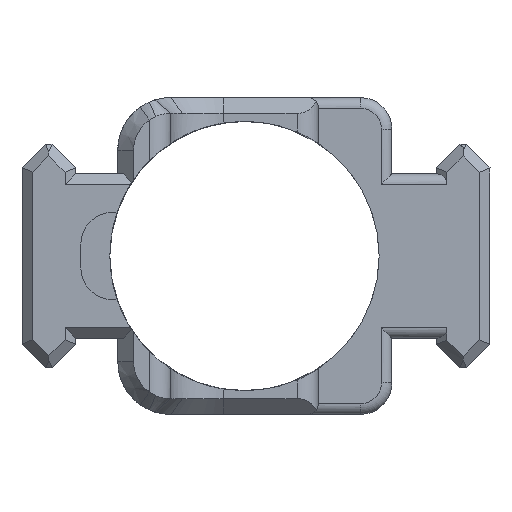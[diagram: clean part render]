
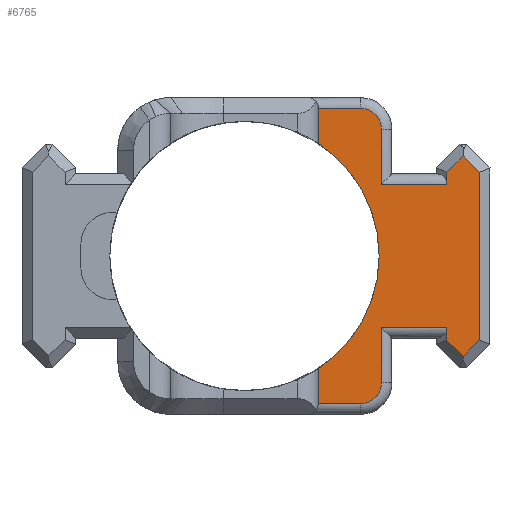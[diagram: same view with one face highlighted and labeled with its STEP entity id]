
A CAD part, left-side view. The second image highlights one B-rep face of the part: STEP entity #6765.
In plain terms, the highlighted planar face has unit normal (-1, 0, 0).
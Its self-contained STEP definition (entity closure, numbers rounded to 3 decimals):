
#152=CIRCLE('',#7203,12.75);
#161=CIRCLE('',#7226,2.);
#162=CIRCLE('',#7227,2.);
#275=FACE_OUTER_BOUND('',#668,.T.);
#668=EDGE_LOOP('',(#4912,#4913,#4914,#4915,#4916,#4917,#4918,#4919,#4920,
#4921,#4922,#4923,#4924,#4925,#4926,#4927,#4928,#4929));
#1260=LINE('',#10404,#2133);
#1261=LINE('',#10408,#2134);
#1264=LINE('',#10424,#2137);
#1268=LINE('',#10437,#2141);
#1269=LINE('',#10439,#2142);
#1270=LINE('',#10441,#2143);
#1271=LINE('',#10443,#2144);
#1272=LINE('',#10445,#2145);
#1273=LINE('',#10447,#2146);
#1274=LINE('',#10449,#2147);
#1275=LINE('',#10451,#2148);
#1276=LINE('',#10453,#2149);
#1277=LINE('',#10455,#2150);
#1278=LINE('',#10457,#2151);
#1279=LINE('',#10460,#2152);
#2133=VECTOR('',#8093,10.);
#2134=VECTOR('',#8098,10.);
#2137=VECTOR('',#8109,10.);
#2141=VECTOR('',#8123,10.);
#2142=VECTOR('',#8124,10.);
#2143=VECTOR('',#8125,10.);
#2144=VECTOR('',#8126,10.);
#2145=VECTOR('',#8127,10.);
#2146=VECTOR('',#8128,10.);
#2147=VECTOR('',#8129,10.);
#2148=VECTOR('',#8130,10.);
#2149=VECTOR('',#8131,10.);
#2150=VECTOR('',#8132,10.);
#2151=VECTOR('',#8133,10.);
#2152=VECTOR('',#8136,10.);
#2971=VERTEX_POINT('',#10185);
#2978=VERTEX_POINT('',#10219);
#2979=VERTEX_POINT('',#10221);
#3006=VERTEX_POINT('',#10406);
#3009=VERTEX_POINT('',#10418);
#3012=VERTEX_POINT('',#10434);
#3013=VERTEX_POINT('',#10436);
#3014=VERTEX_POINT('',#10438);
#3015=VERTEX_POINT('',#10440);
#3016=VERTEX_POINT('',#10442);
#3017=VERTEX_POINT('',#10444);
#3018=VERTEX_POINT('',#10446);
#3019=VERTEX_POINT('',#10448);
#3020=VERTEX_POINT('',#10450);
#3021=VERTEX_POINT('',#10452);
#3022=VERTEX_POINT('',#10454);
#3023=VERTEX_POINT('',#10456);
#3024=VERTEX_POINT('',#10458);
#3669=EDGE_CURVE('',#2979,#2978,#152,.T.);
#3701=EDGE_CURVE('',#2978,#2971,#1260,.T.);
#3703=EDGE_CURVE('',#3006,#2971,#1261,.T.);
#3709=EDGE_CURVE('',#3009,#2979,#1264,.T.);
#3714=EDGE_CURVE('',#3012,#3006,#161,.T.);
#3715=EDGE_CURVE('',#3013,#3012,#1268,.T.);
#3716=EDGE_CURVE('',#3014,#3013,#1269,.T.);
#3717=EDGE_CURVE('',#3015,#3014,#1270,.T.);
#3718=EDGE_CURVE('',#3016,#3015,#1271,.T.);
#3719=EDGE_CURVE('',#3017,#3016,#1272,.T.);
#3720=EDGE_CURVE('',#3018,#3017,#1273,.T.);
#3721=EDGE_CURVE('',#3019,#3018,#1274,.T.);
#3722=EDGE_CURVE('',#3020,#3019,#1275,.T.);
#3723=EDGE_CURVE('',#3021,#3020,#1276,.T.);
#3724=EDGE_CURVE('',#3022,#3021,#1277,.T.);
#3725=EDGE_CURVE('',#3023,#3022,#1278,.T.);
#3726=EDGE_CURVE('',#3024,#3023,#162,.T.);
#3727=EDGE_CURVE('',#3009,#3024,#1279,.T.);
#4912=ORIENTED_EDGE('',*,*,#3669,.T.);
#4913=ORIENTED_EDGE('',*,*,#3701,.T.);
#4914=ORIENTED_EDGE('',*,*,#3703,.F.);
#4915=ORIENTED_EDGE('',*,*,#3714,.F.);
#4916=ORIENTED_EDGE('',*,*,#3715,.F.);
#4917=ORIENTED_EDGE('',*,*,#3716,.F.);
#4918=ORIENTED_EDGE('',*,*,#3717,.F.);
#4919=ORIENTED_EDGE('',*,*,#3718,.F.);
#4920=ORIENTED_EDGE('',*,*,#3719,.F.);
#4921=ORIENTED_EDGE('',*,*,#3720,.F.);
#4922=ORIENTED_EDGE('',*,*,#3721,.F.);
#4923=ORIENTED_EDGE('',*,*,#3722,.F.);
#4924=ORIENTED_EDGE('',*,*,#3723,.F.);
#4925=ORIENTED_EDGE('',*,*,#3724,.F.);
#4926=ORIENTED_EDGE('',*,*,#3725,.F.);
#4927=ORIENTED_EDGE('',*,*,#3726,.F.);
#4928=ORIENTED_EDGE('',*,*,#3727,.F.);
#4929=ORIENTED_EDGE('',*,*,#3709,.T.);
#6403=PLANE('',#7225);
#6765=ADVANCED_FACE('',(#275),#6403,.T.);
#7203=AXIS2_PLACEMENT_3D('',#10222,#8058,#8059);
#7225=AXIS2_PLACEMENT_3D('',#10433,#8119,#8120);
#7226=AXIS2_PLACEMENT_3D('',#10435,#8121,#8122);
#7227=AXIS2_PLACEMENT_3D('',#10459,#8134,#8135);
#8058=DIRECTION('center_axis',(1.,0.,0.));
#8059=DIRECTION('ref_axis',(0.,-1.,0.));
#8093=DIRECTION('',(0.,0.,-1.));
#8098=DIRECTION('',(0.,1.,0.));
#8109=DIRECTION('',(0.,0.,-1.));
#8119=DIRECTION('center_axis',(-1.,0.,0.));
#8120=DIRECTION('ref_axis',(0.,-1.,0.));
#8121=DIRECTION('center_axis',(1.,0.,0.));
#8122=DIRECTION('ref_axis',(0.,-0.707,-0.707));
#8123=DIRECTION('',(0.,0.,-1.));
#8124=DIRECTION('',(0.,1.,0.));
#8125=DIRECTION('',(0.,0.,1.));
#8126=DIRECTION('',(0.,0.707,0.707));
#8127=DIRECTION('',(0.,0.707,-0.707));
#8128=DIRECTION('',(0.,0.,-1.));
#8129=DIRECTION('',(0.,-0.707,-0.707));
#8130=DIRECTION('',(0.,-0.707,0.707));
#8131=DIRECTION('',(0.,0.,1.));
#8132=DIRECTION('',(0.,-1.,0.));
#8133=DIRECTION('',(0.,0.,-1.));
#8134=DIRECTION('center_axis',(1.,0.,0.));
#8135=DIRECTION('ref_axis',(0.,-0.707,0.707));
#8136=DIRECTION('',(0.,-1.,0.));
#10185=CARTESIAN_POINT('',(-1.,86.015,1.));
#10219=CARTESIAN_POINT('',(-1.,86.015,4.334));
#10221=CARTESIAN_POINT('',(-1.,86.015,25.666));
#10222=CARTESIAN_POINT('Origin',(-1.,93.,15.));
#10404=CARTESIAN_POINT('',(-1.,86.015,0.));
#10406=CARTESIAN_POINT('',(-1.,82.03,1.));
#10408=CARTESIAN_POINT('',(-1.,101.5,1.));
#10418=CARTESIAN_POINT('',(-1.,86.015,29.));
#10424=CARTESIAN_POINT('',(-1.,86.015,12.682));
#10433=CARTESIAN_POINT('Origin',(-1.,110.,0.));
#10434=CARTESIAN_POINT('',(-1.,80.03,3.));
#10435=CARTESIAN_POINT('Origin',(-1.,82.03,3.));
#10436=CARTESIAN_POINT('',(-1.,80.03,8.219));
#10437=CARTESIAN_POINT('',(-1.,80.03,-0.187));
#10438=CARTESIAN_POINT('',(-1.,73.827,8.219));
#10439=CARTESIAN_POINT('',(-1.,92.414,8.219));
#10440=CARTESIAN_POINT('',(-1.,73.827,7.001));
#10441=CARTESIAN_POINT('',(-1.,73.827,3.324));
#10442=CARTESIAN_POINT('',(-1.,72.287,5.521));
#10443=CARTESIAN_POINT('',(-1.,81.252,14.486));
#10444=CARTESIAN_POINT('',(-1.,70.747,7.061));
#10445=CARTESIAN_POINT('',(-1.,83.297,-5.488));
#10446=CARTESIAN_POINT('',(-1.,70.747,22.921));
#10447=CARTESIAN_POINT('',(-1.,70.747,3.324));
#10448=CARTESIAN_POINT('',(-1.,72.3,24.474));
#10449=CARTESIAN_POINT('',(-1.,74.684,26.857));
#10450=CARTESIAN_POINT('',(-1.,73.827,22.947));
#10451=CARTESIAN_POINT('',(-1.,87.642,9.132));
#10452=CARTESIAN_POINT('',(-1.,73.827,21.79));
#10453=CARTESIAN_POINT('',(-1.,73.827,11.382));
#10454=CARTESIAN_POINT('',(-1.,80.03,21.79));
#10455=CARTESIAN_POINT('',(-1.,94.535,21.79));
#10456=CARTESIAN_POINT('',(-1.,80.03,27.));
#10457=CARTESIAN_POINT('',(-1.,80.03,-0.187));
#10458=CARTESIAN_POINT('',(-1.,82.03,29.));
#10459=CARTESIAN_POINT('Origin',(-1.,82.03,27.));
#10460=CARTESIAN_POINT('',(-1.,101.5,29.));
